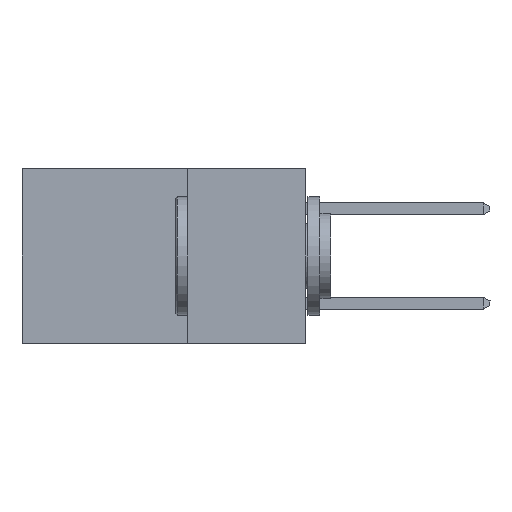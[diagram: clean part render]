
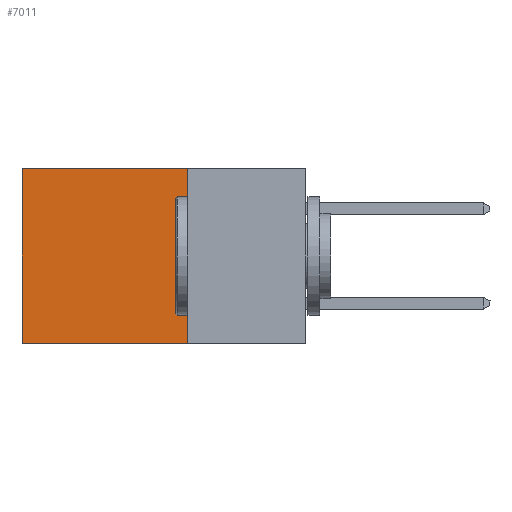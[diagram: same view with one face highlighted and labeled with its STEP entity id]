
A CAD part, left-side view. The second image highlights one B-rep face of the part: STEP entity #7011.
In plain terms, the highlighted planar face has unit normal (-1, 0, 0).
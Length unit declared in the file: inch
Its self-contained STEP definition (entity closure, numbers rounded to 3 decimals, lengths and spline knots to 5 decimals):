
#7 = VECTOR ( 'NONE', #12149, 39.37008 ) ;
#538 = CARTESIAN_POINT ( 'NONE',  ( 0.298, 0.6, -0.37 ) ) ;
#1263 = CARTESIAN_POINT ( 'NONE',  ( 0.298, 0.6, 0. ) ) ;
#1359 = CARTESIAN_POINT ( 'NONE',  ( 0.298, 0.6, 0. ) ) ;
#1769 = ORIENTED_EDGE ( 'NONE', *, *, #11346, .T. ) ;
#1970 = EDGE_CURVE ( 'NONE', #11817, #8012, #3518, .T. ) ;
#2433 = CARTESIAN_POINT ( 'NONE',  ( 0.298, 0.25, -0.37 ) ) ;
#2576 = ORIENTED_EDGE ( 'NONE', *, *, #1970, .T. ) ;
#2625 = CARTESIAN_POINT ( 'NONE',  ( 0.298, 0.25, 0. ) ) ;
#3343 = DIRECTION ( 'NONE',  ( 0., 0., -1. ) ) ;
#3475 = VECTOR ( 'NONE', #3489, 39.37008 ) ;
#3489 = DIRECTION ( 'NONE',  ( 0., 1., 0. ) ) ;
#3518 = LINE ( 'NONE', #1359, #7 ) ;
#4505 = CARTESIAN_POINT ( 'NONE',  ( 0.298, 0.25, 0. ) ) ;
#4862 = VERTEX_POINT ( 'NONE', #5938 ) ;
#5219 = EDGE_LOOP ( 'NONE', ( #2576, #9944, #9864, #1769 ) ) ;
#5535 = CARTESIAN_POINT ( 'NONE',  ( 0.298, 0.25, 0. ) ) ;
#5938 = CARTESIAN_POINT ( 'NONE',  ( 0.298, 0.25, -0.37 ) ) ;
#6233 = LINE ( 'NONE', #4505, #7069 ) ;
#7011 = ADVANCED_FACE ( 'NONE', ( #11221 ), #7983, .F. ) ;
#7069 = VECTOR ( 'NONE', #3343, 39.37008 ) ;
#7983 = PLANE ( 'NONE',  #13229 ) ;
#8012 = VERTEX_POINT ( 'NONE', #538 ) ;
#9093 = EDGE_CURVE ( 'NONE', #4862, #8012, #11664, .T. ) ;
#9159 = DIRECTION ( 'NONE',  ( 0., 1., 0. ) ) ;
#9321 = CARTESIAN_POINT ( 'NONE',  ( 0.298, 0.25, 0. ) ) ;
#9660 = LINE ( 'NONE', #5535, #9838 ) ;
#9797 = VERTEX_POINT ( 'NONE', #9321 ) ;
#9838 = VECTOR ( 'NONE', #9159, 39.37008 ) ;
#9864 = ORIENTED_EDGE ( 'NONE', *, *, #13146, .F. ) ;
#9944 = ORIENTED_EDGE ( 'NONE', *, *, #9093, .F. ) ;
#10118 = DIRECTION ( 'NONE',  ( 1., 0., 0. ) ) ;
#11200 = DIRECTION ( 'NONE',  ( 0., 0., -1. ) ) ;
#11221 = FACE_OUTER_BOUND ( 'NONE', #5219, .T. ) ;
#11346 = EDGE_CURVE ( 'NONE', #9797, #11817, #9660, .T. ) ;
#11664 = LINE ( 'NONE', #2433, #3475 ) ;
#11817 = VERTEX_POINT ( 'NONE', #1263 ) ;
#12149 = DIRECTION ( 'NONE',  ( 0., 0., -1. ) ) ;
#13146 = EDGE_CURVE ( 'NONE', #9797, #4862, #6233, .T. ) ;
#13229 = AXIS2_PLACEMENT_3D ( 'NONE', #2625, #10118, #11200 ) ;
